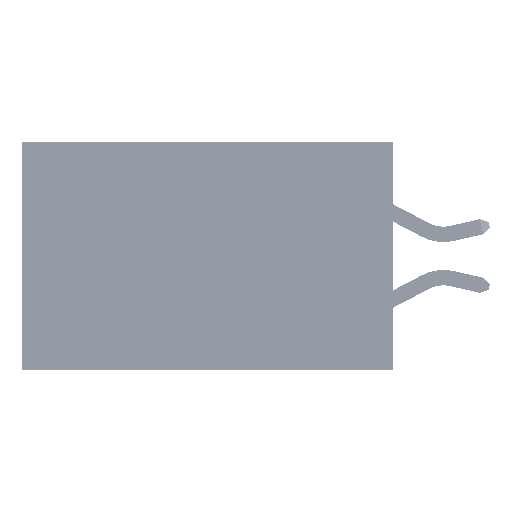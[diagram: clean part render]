
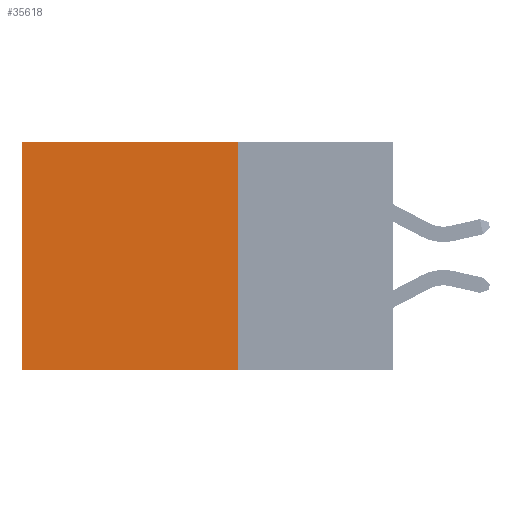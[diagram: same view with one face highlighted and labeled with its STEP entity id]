
A CAD part, left-side view. The second image highlights one B-rep face of the part: STEP entity #35618.
In plain terms, the highlighted planar face has unit normal (-1, 0, 0).
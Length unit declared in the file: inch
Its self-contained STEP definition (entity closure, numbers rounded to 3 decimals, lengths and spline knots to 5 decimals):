
#38 = DIRECTION ( 'NONE',  ( 0., 0., -1. ) ) ;
#3590 = CARTESIAN_POINT ( 'NONE',  ( 0.2875, 0.25, 0. ) ) ;
#3649 = ORIENTED_EDGE ( 'NONE', *, *, #45656, .F. ) ;
#6924 = EDGE_CURVE ( 'NONE', #14546, #21529, #19478, .T. ) ;
#11860 = CARTESIAN_POINT ( 'NONE',  ( 0.2875, 0.6, 0. ) ) ;
#12083 = ORIENTED_EDGE ( 'NONE', *, *, #23236, .T. ) ;
#13566 = CARTESIAN_POINT ( 'NONE',  ( 0.2875, 0.25, 0. ) ) ;
#14546 = VERTEX_POINT ( 'NONE', #13566 ) ;
#15563 = LINE ( 'NONE', #11860, #18597 ) ;
#18597 = VECTOR ( 'NONE', #46838, 39.37008 ) ;
#19478 = LINE ( 'NONE', #36620, #35735 ) ;
#21529 = VERTEX_POINT ( 'NONE', #36070 ) ;
#23020 = CARTESIAN_POINT ( 'NONE',  ( 0.2875, 0.25, -0.37 ) ) ;
#23236 = EDGE_CURVE ( 'NONE', #21529, #30885, #15563, .T. ) ;
#24473 = LINE ( 'NONE', #43728, #31072 ) ;
#26701 = PLANE ( 'NONE',  #49480 ) ;
#27051 = LINE ( 'NONE', #40707, #27618 ) ;
#27618 = VECTOR ( 'NONE', #41373, 39.37008 ) ;
#27670 = FACE_OUTER_BOUND ( 'NONE', #44351, .T. ) ;
#30355 = ORIENTED_EDGE ( 'NONE', *, *, #35986, .F. ) ;
#30573 = DIRECTION ( 'NONE',  ( 1., 0., 0. ) ) ;
#30885 = VERTEX_POINT ( 'NONE', #45238 ) ;
#31072 = VECTOR ( 'NONE', #36106, 39.37008 ) ;
#35618 = ADVANCED_FACE ( 'NONE', ( #27670 ), #26701, .F. ) ;
#35735 = VECTOR ( 'NONE', #48112, 39.37008 ) ;
#35986 = EDGE_CURVE ( 'NONE', #14546, #40881, #27051, .T. ) ;
#36070 = CARTESIAN_POINT ( 'NONE',  ( 0.2875, 0.6, 0. ) ) ;
#36106 = DIRECTION ( 'NONE',  ( 0., 1., 0. ) ) ;
#36620 = CARTESIAN_POINT ( 'NONE',  ( 0.2875, 0.25, 0. ) ) ;
#38645 = ORIENTED_EDGE ( 'NONE', *, *, #6924, .T. ) ;
#40707 = CARTESIAN_POINT ( 'NONE',  ( 0.2875, 0.25, 0. ) ) ;
#40881 = VERTEX_POINT ( 'NONE', #23020 ) ;
#41373 = DIRECTION ( 'NONE',  ( 0., 0., -1. ) ) ;
#43728 = CARTESIAN_POINT ( 'NONE',  ( 0.2875, 0.25, -0.37 ) ) ;
#44351 = EDGE_LOOP ( 'NONE', ( #12083, #3649, #30355, #38645 ) ) ;
#45238 = CARTESIAN_POINT ( 'NONE',  ( 0.2875, 0.6, -0.37 ) ) ;
#45656 = EDGE_CURVE ( 'NONE', #40881, #30885, #24473, .T. ) ;
#46838 = DIRECTION ( 'NONE',  ( 0., 0., -1. ) ) ;
#48112 = DIRECTION ( 'NONE',  ( 0., 1., 0. ) ) ;
#49480 = AXIS2_PLACEMENT_3D ( 'NONE', #3590, #30573, #38 ) ;
